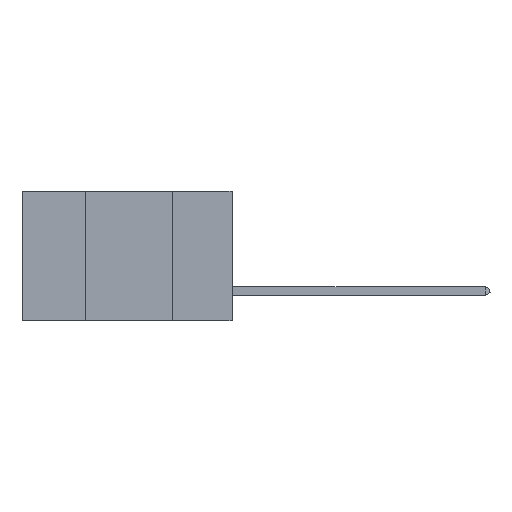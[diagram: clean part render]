
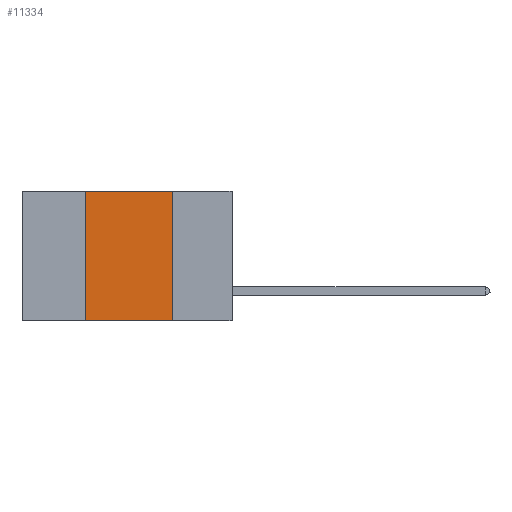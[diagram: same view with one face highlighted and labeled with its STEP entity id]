
A CAD part, left-side view. The second image highlights one B-rep face of the part: STEP entity #11334.
In plain terms, the highlighted planar face has unit normal (-1, 0, 0).
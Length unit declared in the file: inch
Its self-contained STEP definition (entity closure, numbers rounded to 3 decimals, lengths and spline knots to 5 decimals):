
#1311 = DIRECTION ( 'NONE',  ( 0., -1., 0. ) ) ;
#1638 = VECTOR ( 'NONE', #9835, 39.37008 ) ;
#1805 = CARTESIAN_POINT ( 'NONE',  ( 0., 0.17, 0. ) ) ;
#1966 = LINE ( 'NONE', #6881, #13803 ) ;
#2272 = VECTOR ( 'NONE', #7186, 39.37008 ) ;
#2297 = CARTESIAN_POINT ( 'NONE',  ( 0., 0.42, 0. ) ) ;
#2420 = VERTEX_POINT ( 'NONE', #13983 ) ;
#2597 = CARTESIAN_POINT ( 'NONE',  ( 0., 0.42, 0. ) ) ;
#3134 = CARTESIAN_POINT ( 'NONE',  ( 0., 0.6, 0. ) ) ;
#4767 = CARTESIAN_POINT ( 'NONE',  ( 0., 0.17, -0.37 ) ) ;
#4870 = DIRECTION ( 'NONE',  ( 0., 0., 1. ) ) ;
#5301 = EDGE_CURVE ( 'NONE', #2420, #6230, #9423, .T. ) ;
#6230 = VERTEX_POINT ( 'NONE', #2297 ) ;
#6727 = LINE ( 'NONE', #7234, #2272 ) ;
#6881 = CARTESIAN_POINT ( 'NONE',  ( 0., 0.6, -0.37 ) ) ;
#6919 = AXIS2_PLACEMENT_3D ( 'NONE', #3134, #8703, #10755 ) ;
#6955 = LINE ( 'NONE', #7675, #1638 ) ;
#7073 = ORIENTED_EDGE ( 'NONE', *, *, #14151, .F. ) ;
#7186 = DIRECTION ( 'NONE',  ( 0., -1., 0. ) ) ;
#7234 = CARTESIAN_POINT ( 'NONE',  ( 0., 0.6, 0. ) ) ;
#7675 = CARTESIAN_POINT ( 'NONE',  ( 0., 0.17, 0. ) ) ;
#7899 = ORIENTED_EDGE ( 'NONE', *, *, #12034, .T. ) ;
#7926 = VERTEX_POINT ( 'NONE', #4767 ) ;
#8132 = VERTEX_POINT ( 'NONE', #1805 ) ;
#8426 = VECTOR ( 'NONE', #4870, 39.37008 ) ;
#8659 = PLANE ( 'NONE',  #6919 ) ;
#8703 = DIRECTION ( 'NONE',  ( 1., 0., 0. ) ) ;
#9269 = EDGE_LOOP ( 'NONE', ( #13000, #7073, #11127, #7899 ) ) ;
#9423 = LINE ( 'NONE', #2597, #8426 ) ;
#9835 = DIRECTION ( 'NONE',  ( 0., 0., -1. ) ) ;
#10755 = DIRECTION ( 'NONE',  ( 0., 0., -1. ) ) ;
#11127 = ORIENTED_EDGE ( 'NONE', *, *, #5301, .F. ) ;
#11334 = ADVANCED_FACE ( 'NONE', ( #11731 ), #8659, .F. ) ;
#11608 = EDGE_CURVE ( 'NONE', #8132, #7926, #6955, .T. ) ;
#11731 = FACE_OUTER_BOUND ( 'NONE', #9269, .T. ) ;
#12034 = EDGE_CURVE ( 'NONE', #2420, #7926, #1966, .T. ) ;
#13000 = ORIENTED_EDGE ( 'NONE', *, *, #11608, .F. ) ;
#13803 = VECTOR ( 'NONE', #1311, 39.37008 ) ;
#13983 = CARTESIAN_POINT ( 'NONE',  ( 0., 0.42, -0.37 ) ) ;
#14151 = EDGE_CURVE ( 'NONE', #6230, #8132, #6727, .T. ) ;
